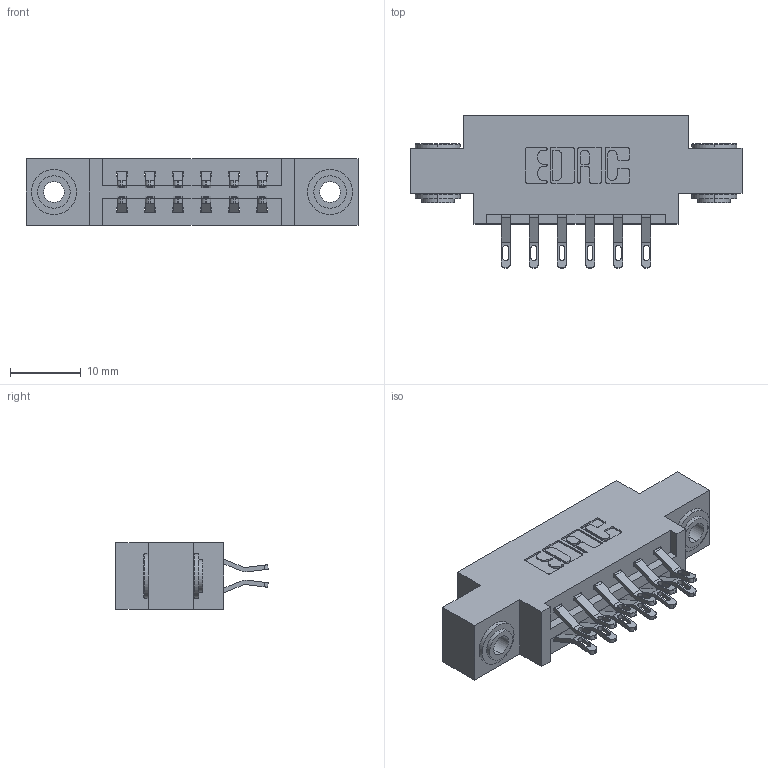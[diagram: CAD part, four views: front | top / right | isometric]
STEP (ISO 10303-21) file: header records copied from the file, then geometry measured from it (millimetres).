
FILE_DESCRIPTION (( 'STEP AP203' ), '1' );
FILE_NAME ('337-012-555-803.STEP', '2019-10-10T16:13:55', ( '' ), ( '' ), 'SwSTEP 2.0', 'SolidWorks 2016', '' );
FILE_SCHEMA (( 'CONFIG_CONTROL_DESIGN' ));
Length unit declared in the file: inch
Products named in the file (4): 337-012-555-803; 345-250-002_345-250-002-102; 345-292-001_555 Tail; 337 Part_0.170 Offset - 0.156 Dia-TH
Assembly tree (15 placements, depth 2):
  337-012-555-803
    337 Part_0.170 Offset - 0.156 Dia-TH
    345-292-001_555 Tail  x12
    345-250-002_345-250-002-102  x2
Bounding box: 46.79 x 21.47 x 9.4 mm (x, y, z)
Volume: 4388.3 mm3; surface area: 5074.7 mm2
Topology: 15 solids, 15 shells, 876 faces, 2667 edges, 1774 vertices
Faces by surface type: plane 516, cylinder 352, cone 8
Entity records: 10416 total; most frequent: CARTESIAN_POINT 1795, ORIENTED_EDGE 1694, DIRECTION 1597, EDGE_CURVE 847, LINE 675, VECTOR 675, VERTEX_POINT 562, AXIS2_PLACEMENT_3D 461
